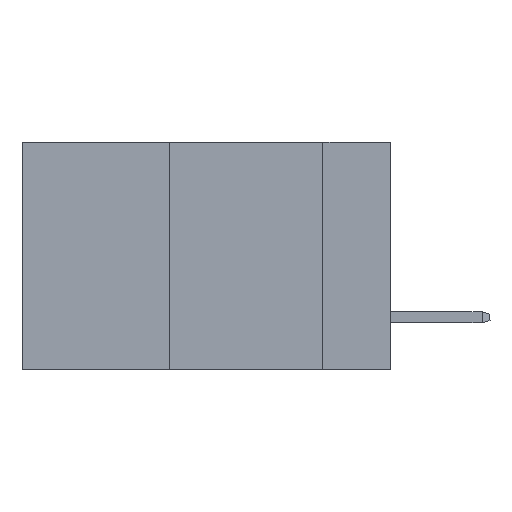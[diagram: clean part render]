
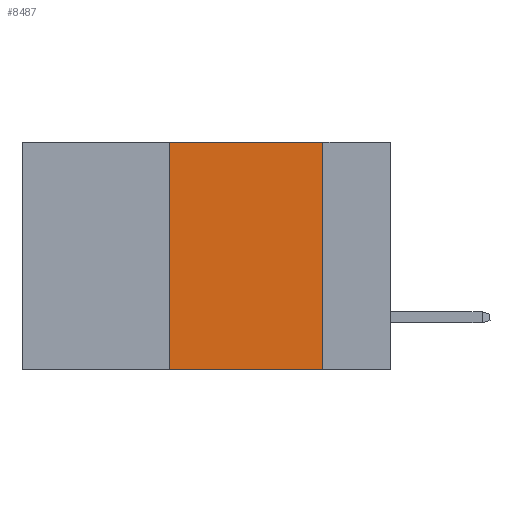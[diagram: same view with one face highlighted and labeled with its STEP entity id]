
A CAD part, left-side view. The second image highlights one B-rep face of the part: STEP entity #8487.
In plain terms, the highlighted planar face has unit normal (-1, 0, 0).
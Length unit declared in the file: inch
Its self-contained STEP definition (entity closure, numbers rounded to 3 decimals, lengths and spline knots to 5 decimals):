
#341 = CARTESIAN_POINT ( 'NONE',  ( 0., 0.11, -0.37 ) ) ;
#402 = CARTESIAN_POINT ( 'NONE',  ( 0., 0.11, 0. ) ) ;
#623 = LINE ( 'NONE', #11938, #16199 ) ;
#775 = VECTOR ( 'NONE', #13494, 39.37008 ) ;
#1212 = DIRECTION ( 'NONE',  ( 0., 0., -1. ) ) ;
#1763 = CARTESIAN_POINT ( 'NONE',  ( 0., 0.36, 0. ) ) ;
#2071 = VECTOR ( 'NONE', #5664, 39.37008 ) ;
#3063 = DIRECTION ( 'NONE',  ( 0., -1., 0. ) ) ;
#4149 = EDGE_LOOP ( 'NONE', ( #8419, #12240, #12672, #16355 ) ) ;
#4162 = FACE_OUTER_BOUND ( 'NONE', #4149, .T. ) ;
#5376 = AXIS2_PLACEMENT_3D ( 'NONE', #12219, #17764, #9413 ) ;
#5664 = DIRECTION ( 'NONE',  ( 0., -1., 0. ) ) ;
#6124 = LINE ( 'NONE', #18379, #2071 ) ;
#8242 = VECTOR ( 'NONE', #1212, 39.37008 ) ;
#8419 = ORIENTED_EDGE ( 'NONE', *, *, #15773, .F. ) ;
#8487 = ADVANCED_FACE ( 'NONE', ( #4162 ), #15048, .F. ) ;
#8749 = CARTESIAN_POINT ( 'NONE',  ( 0., 0.36, -0.37 ) ) ;
#9413 = DIRECTION ( 'NONE',  ( 0., 0., -1. ) ) ;
#9699 = VERTEX_POINT ( 'NONE', #341 ) ;
#10269 = CARTESIAN_POINT ( 'NONE',  ( 0., 0.36, 0. ) ) ;
#11590 = CARTESIAN_POINT ( 'NONE',  ( 0., 0.11, 0. ) ) ;
#11938 = CARTESIAN_POINT ( 'NONE',  ( 0., 0.6, 0. ) ) ;
#12083 = LINE ( 'NONE', #11590, #8242 ) ;
#12219 = CARTESIAN_POINT ( 'NONE',  ( 0., 0.6, 0. ) ) ;
#12240 = ORIENTED_EDGE ( 'NONE', *, *, #12309, .F. ) ;
#12309 = EDGE_CURVE ( 'NONE', #14040, #14887, #623, .T. ) ;
#12641 = LINE ( 'NONE', #1763, #775 ) ;
#12672 = ORIENTED_EDGE ( 'NONE', *, *, #17879, .F. ) ;
#13494 = DIRECTION ( 'NONE',  ( 0., 0., 1. ) ) ;
#14040 = VERTEX_POINT ( 'NONE', #10269 ) ;
#14887 = VERTEX_POINT ( 'NONE', #402 ) ;
#15048 = PLANE ( 'NONE',  #5376 ) ;
#15773 = EDGE_CURVE ( 'NONE', #14887, #9699, #12083, .T. ) ;
#16199 = VECTOR ( 'NONE', #3063, 39.37008 ) ;
#16355 = ORIENTED_EDGE ( 'NONE', *, *, #16470, .T. ) ;
#16470 = EDGE_CURVE ( 'NONE', #17679, #9699, #6124, .T. ) ;
#17679 = VERTEX_POINT ( 'NONE', #8749 ) ;
#17764 = DIRECTION ( 'NONE',  ( 1., 0., 0. ) ) ;
#17879 = EDGE_CURVE ( 'NONE', #17679, #14040, #12641, .T. ) ;
#18379 = CARTESIAN_POINT ( 'NONE',  ( 0., 0.6, -0.37 ) ) ;
